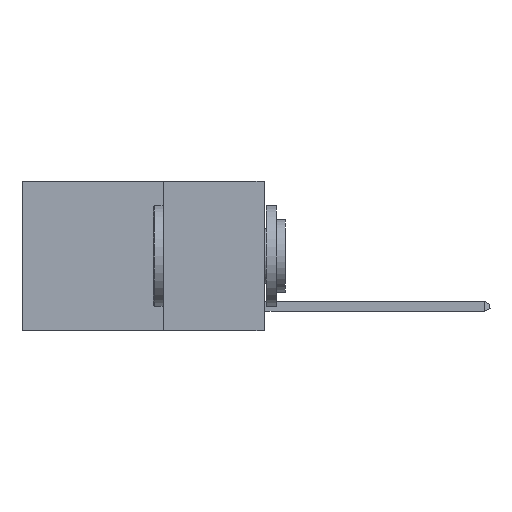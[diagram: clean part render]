
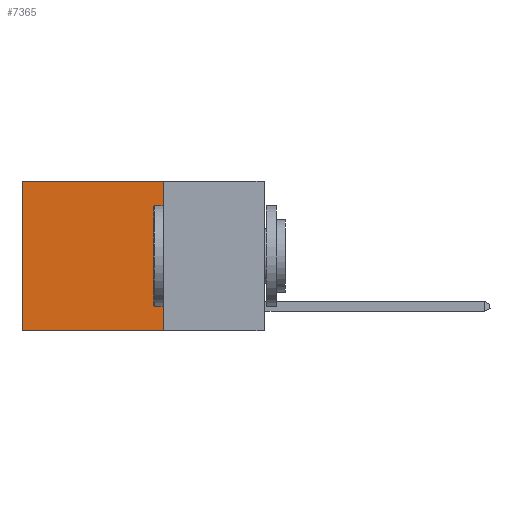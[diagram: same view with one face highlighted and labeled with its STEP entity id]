
A CAD part, left-side view. The second image highlights one B-rep face of the part: STEP entity #7365.
In plain terms, the highlighted planar face has unit normal (-1, 0, 0).
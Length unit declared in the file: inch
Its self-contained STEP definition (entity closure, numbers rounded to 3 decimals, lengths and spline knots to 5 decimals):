
#282 = CARTESIAN_POINT ( 'NONE',  ( 0.2625, 0.25, -0.37 ) ) ;
#475 = CARTESIAN_POINT ( 'NONE',  ( 0.2625, 0.6, 0. ) ) ;
#813 = LINE ( 'NONE', #4449, #5504 ) ;
#1338 = EDGE_CURVE ( 'NONE', #4861, #11787, #813, .T. ) ;
#1641 = CARTESIAN_POINT ( 'NONE',  ( 0.2625, 0.6, 0. ) ) ;
#1763 = DIRECTION ( 'NONE',  ( 0., 0., -1. ) ) ;
#2614 = ORIENTED_EDGE ( 'NONE', *, *, #1338, .T. ) ;
#2758 = CARTESIAN_POINT ( 'NONE',  ( 0.2625, 0.25, 0. ) ) ;
#2922 = EDGE_CURVE ( 'NONE', #10708, #8785, #12056, .T. ) ;
#2936 = CARTESIAN_POINT ( 'NONE',  ( 0.2625, 0.25, -0.37 ) ) ;
#3734 = CARTESIAN_POINT ( 'NONE',  ( 0.2625, 0.6, -0.37 ) ) ;
#4428 = LINE ( 'NONE', #475, #9106 ) ;
#4449 = CARTESIAN_POINT ( 'NONE',  ( 0.2625, 0.25, 0. ) ) ;
#4563 = PLANE ( 'NONE',  #10685 ) ;
#4565 = DIRECTION ( 'NONE',  ( 0., 1., 0. ) ) ;
#4861 = VERTEX_POINT ( 'NONE', #9158 ) ;
#5120 = ORIENTED_EDGE ( 'NONE', *, *, #10381, .T. ) ;
#5380 = DIRECTION ( 'NONE',  ( 1., 0., 0. ) ) ;
#5504 = VECTOR ( 'NONE', #4565, 39.37008 ) ;
#6350 = DIRECTION ( 'NONE',  ( 0., 0., -1. ) ) ;
#7365 = ADVANCED_FACE ( 'NONE', ( #9232 ), #4563, .F. ) ;
#7372 = DIRECTION ( 'NONE',  ( 0., 0., -1. ) ) ;
#8323 = ORIENTED_EDGE ( 'NONE', *, *, #11886, .F. ) ;
#8785 = VERTEX_POINT ( 'NONE', #3734 ) ;
#9086 = DIRECTION ( 'NONE',  ( 0., 1., 0. ) ) ;
#9106 = VECTOR ( 'NONE', #6350, 39.37008 ) ;
#9133 = VECTOR ( 'NONE', #1763, 39.37008 ) ;
#9158 = CARTESIAN_POINT ( 'NONE',  ( 0.2625, 0.25, 0. ) ) ;
#9232 = FACE_OUTER_BOUND ( 'NONE', #10731, .T. ) ;
#9476 = CARTESIAN_POINT ( 'NONE',  ( 0.2625, 0.25, 0. ) ) ;
#10381 = EDGE_CURVE ( 'NONE', #11787, #8785, #4428, .T. ) ;
#10685 = AXIS2_PLACEMENT_3D ( 'NONE', #9476, #5380, #7372 ) ;
#10708 = VERTEX_POINT ( 'NONE', #2936 ) ;
#10731 = EDGE_LOOP ( 'NONE', ( #5120, #11936, #8323, #2614 ) ) ;
#11439 = LINE ( 'NONE', #2758, #9133 ) ;
#11787 = VERTEX_POINT ( 'NONE', #1641 ) ;
#11886 = EDGE_CURVE ( 'NONE', #4861, #10708, #11439, .T. ) ;
#11936 = ORIENTED_EDGE ( 'NONE', *, *, #2922, .F. ) ;
#12056 = LINE ( 'NONE', #282, #12489 ) ;
#12489 = VECTOR ( 'NONE', #9086, 39.37008 ) ;
